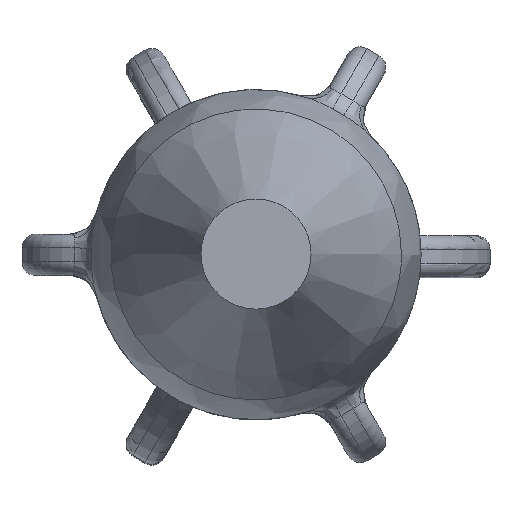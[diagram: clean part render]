
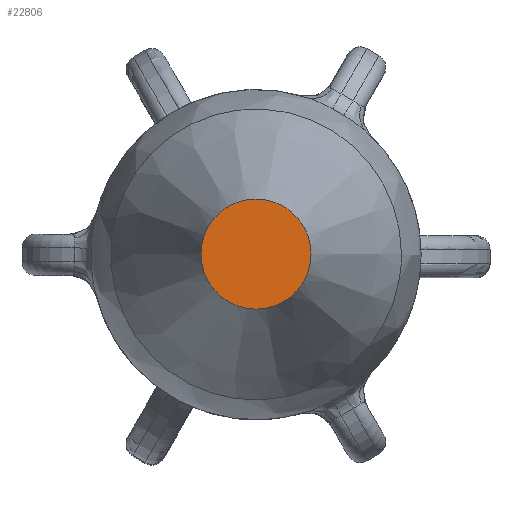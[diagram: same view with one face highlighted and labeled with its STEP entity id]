
A CAD part, top view. The second image highlights one B-rep face of the part: STEP entity #22806.
In plain terms, the highlighted planar face has unit normal (0, 0, 1).
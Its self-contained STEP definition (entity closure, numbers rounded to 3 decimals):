
#19086 = CONICAL_SURFACE('',#19087,12.,0.381);
#19087 = AXIS2_PLACEMENT_3D('',#19088,#19089,#19090);
#19088 = CARTESIAN_POINT('',(0.,0.,110.));
#19089 = DIRECTION('',(-0.,-0.,-1.));
#19090 = DIRECTION('',(1.,0.,0.));
#22565 = VERTEX_POINT('',#22566);
#22566 = CARTESIAN_POINT('',(4.,0.,130.));
#22587 = EDGE_CURVE('',#22565,#22565,#22588,.T.);
#22588 = SURFACE_CURVE('',#22589,(#22594,#22601),.PCURVE_S1.);
#22589 = CIRCLE('',#22590,4.);
#22590 = AXIS2_PLACEMENT_3D('',#22591,#22592,#22593);
#22591 = CARTESIAN_POINT('',(0.,0.,130.));
#22592 = DIRECTION('',(0.,0.,1.));
#22593 = DIRECTION('',(1.,0.,0.));
#22594 = PCURVE('',#19086,#22595);
#22595 = DEFINITIONAL_REPRESENTATION('',(#22596),#22600);
#22596 = LINE('',#22597,#22598);
#22597 = CARTESIAN_POINT('',(-0.,-20.));
#22598 = VECTOR('',#22599,1.);
#22599 = DIRECTION('',(-1.,-0.));
#22600 = ( GEOMETRIC_REPRESENTATION_CONTEXT(2) 
PARAMETRIC_REPRESENTATION_CONTEXT() REPRESENTATION_CONTEXT('2D SPACE',''
  ) );
#22601 = PCURVE('',#22602,#22607);
#22602 = PLANE('',#22603);
#22603 = AXIS2_PLACEMENT_3D('',#22604,#22605,#22606);
#22604 = CARTESIAN_POINT('',(0.,0.,130.));
#22605 = DIRECTION('',(0.,0.,1.));
#22606 = DIRECTION('',(1.,0.,0.));
#22607 = DEFINITIONAL_REPRESENTATION('',(#22608),#22612);
#22608 = CIRCLE('',#22609,4.);
#22609 = AXIS2_PLACEMENT_2D('',#22610,#22611);
#22610 = CARTESIAN_POINT('',(0.,0.));
#22611 = DIRECTION('',(1.,0.));
#22612 = ( GEOMETRIC_REPRESENTATION_CONTEXT(2) 
PARAMETRIC_REPRESENTATION_CONTEXT() REPRESENTATION_CONTEXT('2D SPACE',''
  ) );
#22806 = ADVANCED_FACE('',(#22807),#22602,.T.);
#22807 = FACE_BOUND('',#22808,.T.);
#22808 = EDGE_LOOP('',(#22809));
#22809 = ORIENTED_EDGE('',*,*,#22587,.T.);
